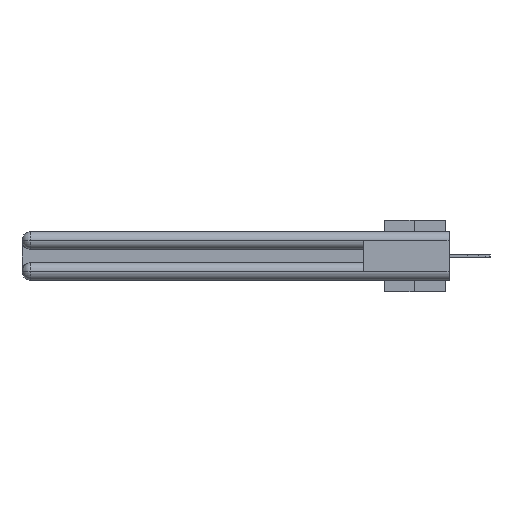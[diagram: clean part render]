
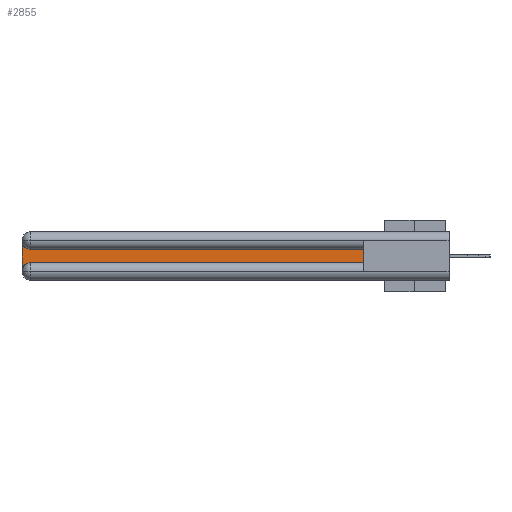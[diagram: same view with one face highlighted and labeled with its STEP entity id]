
A CAD part, left-side view. The second image highlights one B-rep face of the part: STEP entity #2855.
In plain terms, the highlighted planar face has unit normal (-1, 0, 0).
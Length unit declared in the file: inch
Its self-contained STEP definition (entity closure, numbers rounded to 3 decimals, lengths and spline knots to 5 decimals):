
#880 = CARTESIAN_POINT ( 'NONE',  ( 0.075, 0.6, -0.1225 ) ) ;
#1675 = CARTESIAN_POINT ( 'NONE',  ( 0.075, 0.6, -0.2175 ) ) ;
#1756 = CARTESIAN_POINT ( 'NONE',  ( 0.075, 0.6, -0.2175 ) ) ;
#2305 = ORIENTED_EDGE ( 'NONE', *, *, #28435, .T. ) ;
#2855 = ADVANCED_FACE ( 'NONE', ( #17305 ), #23567, .F. ) ;
#3080 = CARTESIAN_POINT ( 'NONE',  ( 0.075, 3., -0.2175 ) ) ;
#3436 = DIRECTION ( 'NONE',  ( 1., 0., 0. ) ) ;
#4547 = DIRECTION ( 'NONE',  ( 0., 0., 1. ) ) ;
#4717 = LINE ( 'NONE', #23980, #31484 ) ;
#4746 = CIRCLE ( 'NONE', #33641, 0.06 ) ;
#5253 = CARTESIAN_POINT ( 'NONE',  ( 0.075, 2.94, -0.2175 ) ) ;
#5281 = DIRECTION ( 'NONE',  ( 0., 1., 0. ) ) ;
#7417 = CARTESIAN_POINT ( 'NONE',  ( 0.075, 3., -0.1225 ) ) ;
#7773 = ORIENTED_EDGE ( 'NONE', *, *, #16289, .T. ) ;
#7935 = VECTOR ( 'NONE', #5281, 39.37008 ) ;
#9198 = LINE ( 'NONE', #1756, #22551 ) ;
#9387 = EDGE_CURVE ( 'NONE', #14810, #27336, #29220, .T. ) ;
#9698 = EDGE_LOOP ( 'NONE', ( #9932, #12405, #2305, #27056, #14384, #7773 ) ) ;
#9932 = ORIENTED_EDGE ( 'NONE', *, *, #9387, .T. ) ;
#10040 = EDGE_CURVE ( 'NONE', #27336, #24030, #22515, .T. ) ;
#10303 = DIRECTION ( 'NONE',  ( 0., 0., -1. ) ) ;
#11936 = EDGE_CURVE ( 'NONE', #21730, #26500, #4746, .T. ) ;
#12394 = EDGE_CURVE ( 'NONE', #26500, #27463, #4717, .T. ) ;
#12405 = ORIENTED_EDGE ( 'NONE', *, *, #10040, .T. ) ;
#14384 = ORIENTED_EDGE ( 'NONE', *, *, #12394, .T. ) ;
#14707 = CARTESIAN_POINT ( 'NONE',  ( 0.075, 2.94, -0.1225 ) ) ;
#14810 = VERTEX_POINT ( 'NONE', #880 ) ;
#16005 = DIRECTION ( 'NONE',  ( 1., 0., 0. ) ) ;
#16289 = EDGE_CURVE ( 'NONE', #27463, #14810, #9198, .T. ) ;
#17305 = FACE_OUTER_BOUND ( 'NONE', #9698, .T. ) ;
#18712 = CARTESIAN_POINT ( 'NONE',  ( 0.075, 3., -0.2775 ) ) ;
#19250 = DIRECTION ( 'NONE',  ( 0., 0., -1. ) ) ;
#19587 = CARTESIAN_POINT ( 'NONE',  ( 0.075, 2.94, -0.2775 ) ) ;
#21318 = DIRECTION ( 'NONE',  ( 0., -1., 0. ) ) ;
#21367 = CARTESIAN_POINT ( 'NONE',  ( 0.075, 0.6, -0.1225 ) ) ;
#21730 = VERTEX_POINT ( 'NONE', #18712 ) ;
#22257 = DIRECTION ( 'NONE',  ( 0., 0., -1. ) ) ;
#22515 = CIRCLE ( 'NONE', #27611, 0.06 ) ;
#22551 = VECTOR ( 'NONE', #4547, 39.37008 ) ;
#23567 = PLANE ( 'NONE',  #27014 ) ;
#23980 = CARTESIAN_POINT ( 'NONE',  ( 0.075, 0.6, -0.2175 ) ) ;
#24030 = VERTEX_POINT ( 'NONE', #29743 ) ;
#25944 = VECTOR ( 'NONE', #19250, 39.37008 ) ;
#26246 = DIRECTION ( 'NONE',  ( 1., 0., 0. ) ) ;
#26500 = VERTEX_POINT ( 'NONE', #5253 ) ;
#26789 = LINE ( 'NONE', #3080, #25944 ) ;
#27014 = AXIS2_PLACEMENT_3D ( 'NONE', #7417, #26246, #10303 ) ;
#27056 = ORIENTED_EDGE ( 'NONE', *, *, #11936, .T. ) ;
#27336 = VERTEX_POINT ( 'NONE', #14707 ) ;
#27463 = VERTEX_POINT ( 'NONE', #1675 ) ;
#27611 = AXIS2_PLACEMENT_3D ( 'NONE', #31861, #16005, #34480 ) ;
#28435 = EDGE_CURVE ( 'NONE', #24030, #21730, #26789, .T. ) ;
#29220 = LINE ( 'NONE', #21367, #7935 ) ;
#29743 = CARTESIAN_POINT ( 'NONE',  ( 0.075, 3., -0.0625 ) ) ;
#31484 = VECTOR ( 'NONE', #21318, 39.37008 ) ;
#31861 = CARTESIAN_POINT ( 'NONE',  ( 0.075, 2.94, -0.0625 ) ) ;
#33641 = AXIS2_PLACEMENT_3D ( 'NONE', #19587, #3436, #22257 ) ;
#34480 = DIRECTION ( 'NONE',  ( 0., 0., -1. ) ) ;
